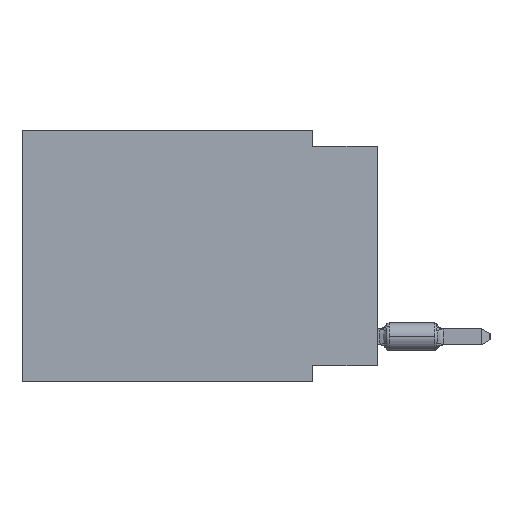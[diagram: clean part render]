
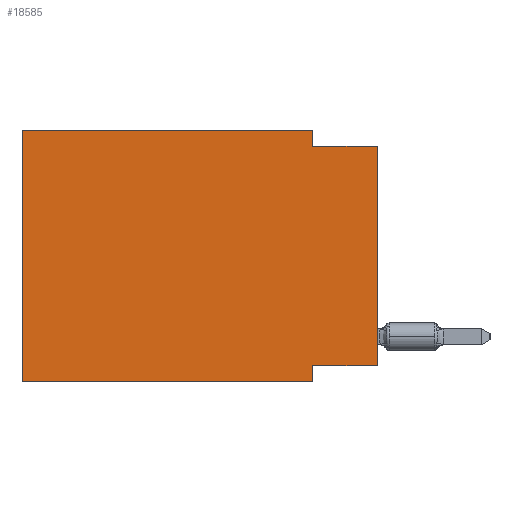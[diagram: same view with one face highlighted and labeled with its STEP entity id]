
A CAD part, left-side view. The second image highlights one B-rep face of the part: STEP entity #18585.
In plain terms, the highlighted planar face has unit normal (-1, 0, 0).
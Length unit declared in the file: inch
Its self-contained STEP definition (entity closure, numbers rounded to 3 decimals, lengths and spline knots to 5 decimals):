
#1185 = VECTOR ( 'NONE', #42960, 39.37008 ) ;
#1272 = DIRECTION ( 'NONE',  ( 1., 0., 0. ) ) ;
#1444 = EDGE_CURVE ( 'NONE', #48291, #2500, #36652, .T. ) ;
#2314 = CARTESIAN_POINT ( 'NONE',  ( 0., 0., -0.025 ) ) ;
#2500 = VERTEX_POINT ( 'NONE', #48461 ) ;
#2934 = AXIS2_PLACEMENT_3D ( 'NONE', #10025, #1272, #37535 ) ;
#3068 = CARTESIAN_POINT ( 'NONE',  ( 0., 0.55, -0.39 ) ) ;
#3741 = VERTEX_POINT ( 'NONE', #14438 ) ;
#3928 = EDGE_LOOP ( 'NONE', ( #20431, #54762, #46401, #46748, #16287, #10848, #25693, #27573 ) ) ;
#5508 = LINE ( 'NONE', #28880, #22013 ) ;
#5802 = DIRECTION ( 'NONE',  ( 0., -1., 0. ) ) ;
#5902 = VERTEX_POINT ( 'NONE', #51375 ) ;
#6681 = LINE ( 'NONE', #2314, #13219 ) ;
#6800 = EDGE_CURVE ( 'NONE', #2500, #9290, #6681, .T. ) ;
#8555 = CARTESIAN_POINT ( 'NONE',  ( 0., 0.55, 0. ) ) ;
#9290 = VERTEX_POINT ( 'NONE', #52766 ) ;
#9613 = CARTESIAN_POINT ( 'NONE',  ( 0., 0., -0.365 ) ) ;
#10025 = CARTESIAN_POINT ( 'NONE',  ( 0., 0.55, 0. ) ) ;
#10848 = ORIENTED_EDGE ( 'NONE', *, *, #43711, .T. ) ;
#13048 = CARTESIAN_POINT ( 'NONE',  ( 0., 0.1, 0. ) ) ;
#13219 = VECTOR ( 'NONE', #15177, 39.37008 ) ;
#14007 = LINE ( 'NONE', #32441, #38126 ) ;
#14411 = DIRECTION ( 'NONE',  ( 0., 0., -1. ) ) ;
#14438 = CARTESIAN_POINT ( 'NONE',  ( 0., 0.1, -0.39 ) ) ;
#15177 = DIRECTION ( 'NONE',  ( 0., -1., 0. ) ) ;
#16223 = DIRECTION ( 'NONE',  ( 0., 0., 1. ) ) ;
#16287 = ORIENTED_EDGE ( 'NONE', *, *, #18343, .F. ) ;
#17136 = DIRECTION ( 'NONE',  ( 0., 1., 0. ) ) ;
#18343 = EDGE_CURVE ( 'NONE', #47566, #27744, #39079, .T. ) ;
#18585 = ADVANCED_FACE ( 'NONE', ( #30857 ), #48767, .F. ) ;
#18658 = VECTOR ( 'NONE', #17136, 39.37008 ) ;
#19436 = EDGE_CURVE ( 'NONE', #5902, #3741, #34716, .T. ) ;
#20431 = ORIENTED_EDGE ( 'NONE', *, *, #48075, .T. ) ;
#21174 = CARTESIAN_POINT ( 'NONE',  ( 0., 0.55, 0. ) ) ;
#21629 = VECTOR ( 'NONE', #16223, 39.37008 ) ;
#22013 = VECTOR ( 'NONE', #5802, 39.37008 ) ;
#23882 = EDGE_CURVE ( 'NONE', #27744, #48291, #34381, .T. ) ;
#25343 = CARTESIAN_POINT ( 'NONE',  ( 0., 0., -0.365 ) ) ;
#25693 = ORIENTED_EDGE ( 'NONE', *, *, #19436, .F. ) ;
#27573 = ORIENTED_EDGE ( 'NONE', *, *, #31947, .F. ) ;
#27744 = VERTEX_POINT ( 'NONE', #8555 ) ;
#28880 = CARTESIAN_POINT ( 'NONE',  ( 0., 0.55, -0.39 ) ) ;
#29166 = CARTESIAN_POINT ( 'NONE',  ( 0., 0.1, -0.39 ) ) ;
#29732 = LINE ( 'NONE', #25343, #18658 ) ;
#30857 = FACE_OUTER_BOUND ( 'NONE', #3928, .T. ) ;
#31586 = DIRECTION ( 'NONE',  ( 0., 0., 1. ) ) ;
#31947 = EDGE_CURVE ( 'NONE', #50195, #5902, #29732, .T. ) ;
#32441 = CARTESIAN_POINT ( 'NONE',  ( 0., 0., 0. ) ) ;
#34381 = LINE ( 'NONE', #52312, #50044 ) ;
#34716 = LINE ( 'NONE', #29166, #1185 ) ;
#36652 = LINE ( 'NONE', #54605, #55850 ) ;
#37535 = DIRECTION ( 'NONE',  ( 0., 0., -1. ) ) ;
#38126 = VECTOR ( 'NONE', #31586, 39.37008 ) ;
#39079 = LINE ( 'NONE', #21174, #21629 ) ;
#42960 = DIRECTION ( 'NONE',  ( 0., 0., -1. ) ) ;
#43711 = EDGE_CURVE ( 'NONE', #47566, #3741, #5508, .T. ) ;
#46401 = ORIENTED_EDGE ( 'NONE', *, *, #1444, .F. ) ;
#46748 = ORIENTED_EDGE ( 'NONE', *, *, #23882, .F. ) ;
#47566 = VERTEX_POINT ( 'NONE', #3068 ) ;
#47894 = DIRECTION ( 'NONE',  ( 0., -1., 0. ) ) ;
#48075 = EDGE_CURVE ( 'NONE', #50195, #9290, #14007, .T. ) ;
#48291 = VERTEX_POINT ( 'NONE', #13048 ) ;
#48461 = CARTESIAN_POINT ( 'NONE',  ( 0., 0.1, -0.025 ) ) ;
#48767 = PLANE ( 'NONE',  #2934 ) ;
#50044 = VECTOR ( 'NONE', #47894, 39.37008 ) ;
#50195 = VERTEX_POINT ( 'NONE', #9613 ) ;
#51375 = CARTESIAN_POINT ( 'NONE',  ( 0., 0.1, -0.365 ) ) ;
#52312 = CARTESIAN_POINT ( 'NONE',  ( 0., 0.55, 0. ) ) ;
#52766 = CARTESIAN_POINT ( 'NONE',  ( 0., 0., -0.025 ) ) ;
#54605 = CARTESIAN_POINT ( 'NONE',  ( 0., 0.1, 0. ) ) ;
#54762 = ORIENTED_EDGE ( 'NONE', *, *, #6800, .F. ) ;
#55850 = VECTOR ( 'NONE', #14411, 39.37008 ) ;
